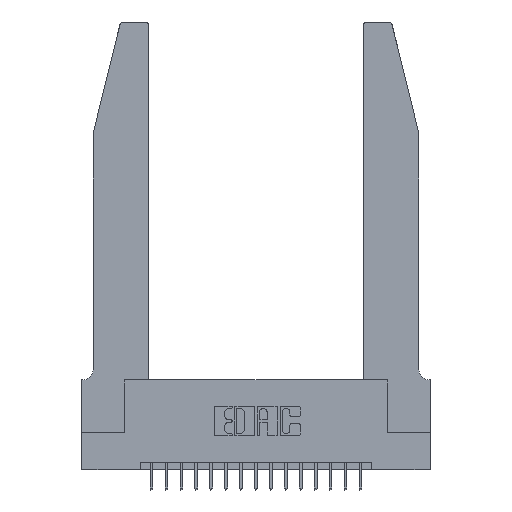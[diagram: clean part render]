
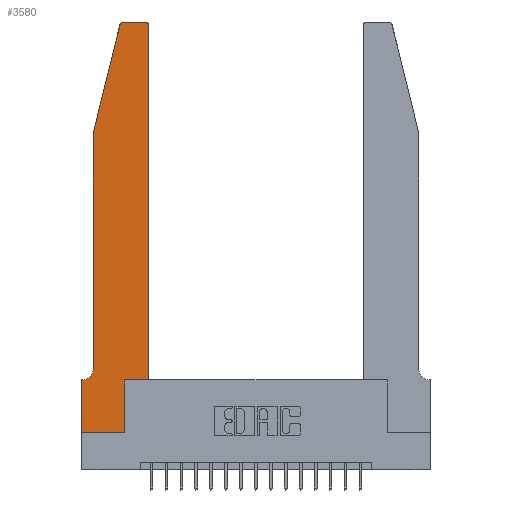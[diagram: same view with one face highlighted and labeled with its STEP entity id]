
A CAD part, top view. The second image highlights one B-rep face of the part: STEP entity #3580.
In plain terms, the highlighted planar face has unit normal (0, 0, 1).
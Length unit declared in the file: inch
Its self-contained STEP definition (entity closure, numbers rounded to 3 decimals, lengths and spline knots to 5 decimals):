
#2 = CARTESIAN_POINT ( 'NONE',  ( 0., 0., 0.37 ) ) ;
#411 = ORIENTED_EDGE ( 'NONE', *, *, #8250, .T. ) ;
#537 = LINE ( 'NONE', #4852, #8776 ) ;
#717 = AXIS2_PLACEMENT_3D ( 'NONE', #7866, #1396, #20034 ) ;
#804 = EDGE_CURVE ( 'NONE', #13767, #19635, #6870, .T. ) ;
#1284 = PLANE ( 'NONE',  #717 ) ;
#1396 = DIRECTION ( 'NONE',  ( 0., 0., 1. ) ) ;
#1399 = CIRCLE ( 'NONE', #12879, 0.03 ) ;
#2244 = DIRECTION ( 'NONE',  ( -1., 0., 0. ) ) ;
#2331 = CARTESIAN_POINT ( 'NONE',  ( 0.284, 2.75, 0.37 ) ) ;
#2460 = LINE ( 'NONE', #15198, #16359 ) ;
#2571 = DIRECTION ( 'NONE',  ( 0., -1., 0. ) ) ;
#2835 = FACE_OUTER_BOUND ( 'NONE', #5091, .T. ) ;
#2911 = VERTEX_POINT ( 'NONE', #4619 ) ;
#3060 = ORIENTED_EDGE ( 'NONE', *, *, #19891, .T. ) ;
#3113 = DIRECTION ( 'NONE',  ( 0., -1., 0. ) ) ;
#3119 = VERTEX_POINT ( 'NONE', #4408 ) ;
#3246 = LINE ( 'NONE', #9312, #13531 ) ;
#3294 = VERTEX_POINT ( 'NONE', #18367 ) ;
#3314 = DIRECTION ( 'NONE',  ( -0.239, -0.971, 0. ) ) ;
#3434 = ORIENTED_EDGE ( 'NONE', *, *, #8450, .T. ) ;
#3580 = ADVANCED_FACE ( 'NONE', ( #2835 ), #1284, .T. ) ;
#3793 = VECTOR ( 'NONE', #4902, 39.37008 ) ;
#3976 = DIRECTION ( 'NONE',  ( -1., 0., 0. ) ) ;
#4240 = CARTESIAN_POINT ( 'NONE',  ( 0.0755, 2., 0.37 ) ) ;
#4311 = DIRECTION ( 'NONE',  ( 1., 0., 0. ) ) ;
#4408 = CARTESIAN_POINT ( 'NONE',  ( 0.4505, 2.72, 0.37 ) ) ;
#4419 = ORIENTED_EDGE ( 'NONE', *, *, #15846, .T. ) ;
#4529 = CARTESIAN_POINT ( 'NONE',  ( 0.25487, 2.72718, 0.37 ) ) ;
#4541 = CARTESIAN_POINT ( 'NONE',  ( 0.2865, 0., 0.37 ) ) ;
#4619 = CARTESIAN_POINT ( 'NONE',  ( 0.4505, 0.35, 0.37 ) ) ;
#4852 = CARTESIAN_POINT ( 'NONE',  ( 0.0755, 2., 0.37 ) ) ;
#4902 = DIRECTION ( 'NONE',  ( 0., 1., 0. ) ) ;
#5091 = EDGE_LOOP ( 'NONE', ( #17829, #411, #3434, #4419, #17466, #16722, #8181, #20065, #10878, #19870, #3060, #12202 ) ) ;
#5836 = DIRECTION ( 'NONE',  ( 0., 0., 1. ) ) ;
#6074 = EDGE_CURVE ( 'NONE', #3119, #3294, #1399, .T. ) ;
#6095 = EDGE_CURVE ( 'NONE', #19635, #18037, #17140, .T. ) ;
#6099 = DIRECTION ( 'NONE',  ( 0., 0., 1. ) ) ;
#6456 = EDGE_CURVE ( 'NONE', #10058, #13767, #18739, .T. ) ;
#6651 = VECTOR ( 'NONE', #3113, 39.37008 ) ;
#6870 = LINE ( 'NONE', #16290, #13458 ) ;
#7553 = CARTESIAN_POINT ( 'NONE',  ( 0., 0.35, 0.37 ) ) ;
#7704 = CARTESIAN_POINT ( 'NONE',  ( 0.0755, 2., 0.37 ) ) ;
#7866 = CARTESIAN_POINT ( 'NONE',  ( 0., 0.35, 0.37 ) ) ;
#8135 = CIRCLE ( 'NONE', #8829, 0.03 ) ;
#8181 = ORIENTED_EDGE ( 'NONE', *, *, #6095, .T. ) ;
#8250 = EDGE_CURVE ( 'NONE', #12033, #11776, #8135, .T. ) ;
#8450 = EDGE_CURVE ( 'NONE', #11776, #11738, #537, .T. ) ;
#8573 = LINE ( 'NONE', #15143, #15981 ) ;
#8776 = VECTOR ( 'NONE', #3314, 39.37008 ) ;
#8799 = EDGE_CURVE ( 'NONE', #3294, #12033, #8573, .T. ) ;
#8829 = AXIS2_PLACEMENT_3D ( 'NONE', #19656, #5836, #4311 ) ;
#9105 = VERTEX_POINT ( 'NONE', #4541 ) ;
#9312 = CARTESIAN_POINT ( 'NONE',  ( 0., 0., 0.37 ) ) ;
#9520 = CARTESIAN_POINT ( 'NONE',  ( 0.2865, 0.35, 0.37 ) ) ;
#9600 = DIRECTION ( 'NONE',  ( 0., 1., 0. ) ) ;
#10058 = VERTEX_POINT ( 'NONE', #19755 ) ;
#10359 = LINE ( 'NONE', #4240, #13614 ) ;
#10396 = DIRECTION ( 'NONE',  ( 0., 0., -1. ) ) ;
#10505 = EDGE_CURVE ( 'NONE', #11639, #2911, #2460, .T. ) ;
#10789 = CARTESIAN_POINT ( 'NONE',  ( 0.4205, 2.72, 0.37 ) ) ;
#10878 = ORIENTED_EDGE ( 'NONE', *, *, #17822, .T. ) ;
#11086 = CARTESIAN_POINT ( 'NONE',  ( 0.0055, 0.42, 0.37 ) ) ;
#11328 = LINE ( 'NONE', #19112, #18117 ) ;
#11639 = VERTEX_POINT ( 'NONE', #14876 ) ;
#11738 = VERTEX_POINT ( 'NONE', #7704 ) ;
#11776 = VERTEX_POINT ( 'NONE', #4529 ) ;
#12033 = VERTEX_POINT ( 'NONE', #2331 ) ;
#12202 = ORIENTED_EDGE ( 'NONE', *, *, #6074, .T. ) ;
#12351 = DIRECTION ( 'NONE',  ( 1., 0., 0. ) ) ;
#12572 = AXIS2_PLACEMENT_3D ( 'NONE', #11086, #10396, #16650 ) ;
#12879 = AXIS2_PLACEMENT_3D ( 'NONE', #10789, #6099, #12351 ) ;
#13458 = VECTOR ( 'NONE', #2244, 39.37008 ) ;
#13520 = EDGE_CURVE ( 'NONE', #18037, #9105, #3246, .T. ) ;
#13531 = VECTOR ( 'NONE', #15575, 39.37008 ) ;
#13614 = VECTOR ( 'NONE', #2571, 39.37008 ) ;
#13725 = CARTESIAN_POINT ( 'NONE',  ( 0., 0., 0.37 ) ) ;
#13767 = VERTEX_POINT ( 'NONE', #14424 ) ;
#13956 = LINE ( 'NONE', #9520, #3793 ) ;
#14424 = CARTESIAN_POINT ( 'NONE',  ( 0.0055, 0.35, 0.37 ) ) ;
#14876 = CARTESIAN_POINT ( 'NONE',  ( 0.2865, 0.35, 0.37 ) ) ;
#15143 = CARTESIAN_POINT ( 'NONE',  ( 0.2605, 2.75, 0.37 ) ) ;
#15198 = CARTESIAN_POINT ( 'NONE',  ( 0.4505, 0.35, 0.37 ) ) ;
#15575 = DIRECTION ( 'NONE',  ( 1., 0., 0. ) ) ;
#15846 = EDGE_CURVE ( 'NONE', #11738, #10058, #10359, .T. ) ;
#15981 = VECTOR ( 'NONE', #3976, 39.37008 ) ;
#16290 = CARTESIAN_POINT ( 'NONE',  ( 0.0755, 0.35, 0.37 ) ) ;
#16359 = VECTOR ( 'NONE', #16599, 39.37008 ) ;
#16599 = DIRECTION ( 'NONE',  ( 1., 0., 0. ) ) ;
#16650 = DIRECTION ( 'NONE',  ( -1., 0., 0. ) ) ;
#16722 = ORIENTED_EDGE ( 'NONE', *, *, #804, .T. ) ;
#17140 = LINE ( 'NONE', #2, #6651 ) ;
#17466 = ORIENTED_EDGE ( 'NONE', *, *, #6456, .T. ) ;
#17822 = EDGE_CURVE ( 'NONE', #9105, #11639, #13956, .T. ) ;
#17829 = ORIENTED_EDGE ( 'NONE', *, *, #8799, .T. ) ;
#18037 = VERTEX_POINT ( 'NONE', #13725 ) ;
#18117 = VECTOR ( 'NONE', #9600, 39.37008 ) ;
#18367 = CARTESIAN_POINT ( 'NONE',  ( 0.4205, 2.75, 0.37 ) ) ;
#18739 = CIRCLE ( 'NONE', #12572, 0.07 ) ;
#19112 = CARTESIAN_POINT ( 'NONE',  ( 0.4505, 0.35, 0.37 ) ) ;
#19635 = VERTEX_POINT ( 'NONE', #7553 ) ;
#19656 = CARTESIAN_POINT ( 'NONE',  ( 0.284, 2.72, 0.37 ) ) ;
#19755 = CARTESIAN_POINT ( 'NONE',  ( 0.0755, 0.42, 0.37 ) ) ;
#19870 = ORIENTED_EDGE ( 'NONE', *, *, #10505, .T. ) ;
#19891 = EDGE_CURVE ( 'NONE', #2911, #3119, #11328, .T. ) ;
#20034 = DIRECTION ( 'NONE',  ( 1., 0., 0. ) ) ;
#20065 = ORIENTED_EDGE ( 'NONE', *, *, #13520, .T. ) ;
